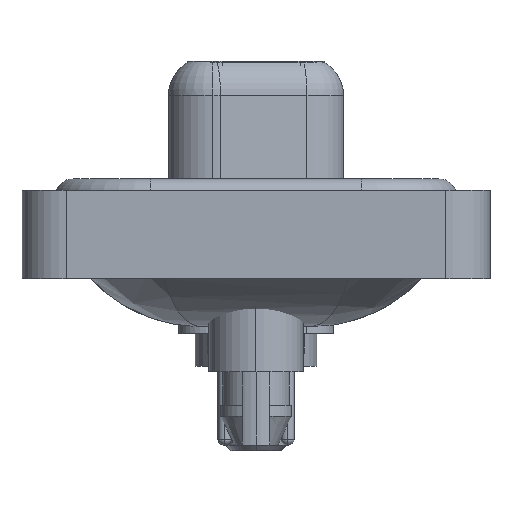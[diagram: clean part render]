
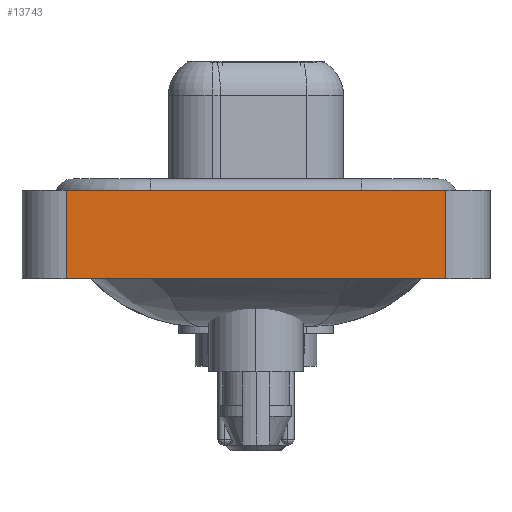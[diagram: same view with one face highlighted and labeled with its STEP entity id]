
A CAD part, left-side view. The second image highlights one B-rep face of the part: STEP entity #13743.
In plain terms, the highlighted planar face has unit normal (-1, 0, 0).
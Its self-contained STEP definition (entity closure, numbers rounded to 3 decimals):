
#519 = CARTESIAN_POINT ( 'NONE',  ( -7.25, -8.55, -3.6 ) ) ;
#941 = DIRECTION ( 'NONE',  ( 0., -1., 0. ) ) ;
#1468 = CARTESIAN_POINT ( 'NONE',  ( -7.25, -8.55, -3.6 ) ) ;
#1543 = EDGE_LOOP ( 'NONE', ( #17771, #7898, #10670, #3893 ) ) ;
#1933 = CARTESIAN_POINT ( 'NONE',  ( -7.25, -8.55, 0.4 ) ) ;
#3010 = EDGE_CURVE ( 'NONE', #9094, #14878, #14602, .T. ) ;
#3022 = AXIS2_PLACEMENT_3D ( 'NONE', #519, #16565, #19919 ) ;
#3397 = VECTOR ( 'NONE', #9768, 1000. ) ;
#3559 = PLANE ( 'NONE',  #3022 ) ;
#3672 = CARTESIAN_POINT ( 'NONE',  ( -7.25, -8.55, -3.6 ) ) ;
#3893 = ORIENTED_EDGE ( 'NONE', *, *, #6115, .T. ) ;
#4909 = LINE ( 'NONE', #1468, #3397 ) ;
#5332 = EDGE_CURVE ( 'NONE', #20415, #6546, #4909, .T. ) ;
#6093 = EDGE_CURVE ( 'NONE', #14878, #6546, #12459, .T. ) ;
#6115 = EDGE_CURVE ( 'NONE', #9094, #20415, #18401, .T. ) ;
#6188 = VECTOR ( 'NONE', #14391, 1000. ) ;
#6546 = VERTEX_POINT ( 'NONE', #15662 ) ;
#7898 = ORIENTED_EDGE ( 'NONE', *, *, #6093, .F. ) ;
#9094 = VERTEX_POINT ( 'NONE', #14737 ) ;
#9768 = DIRECTION ( 'NONE',  ( 0., 0., 1. ) ) ;
#10670 = ORIENTED_EDGE ( 'NONE', *, *, #3010, .F. ) ;
#12459 = LINE ( 'NONE', #1933, #17845 ) ;
#13743 = ADVANCED_FACE ( 'NONE', ( #19805 ), #3559, .T. ) ;
#14391 = DIRECTION ( 'NONE',  ( 0., -1., 0. ) ) ;
#14602 = LINE ( 'NONE', #16230, #18482 ) ;
#14737 = CARTESIAN_POINT ( 'NONE',  ( -7.25, 8.55, -3.6 ) ) ;
#14878 = VERTEX_POINT ( 'NONE', #21036 ) ;
#15662 = CARTESIAN_POINT ( 'NONE',  ( -7.25, -8.55, 0.4 ) ) ;
#16230 = CARTESIAN_POINT ( 'NONE',  ( -7.25, 8.55, -3.6 ) ) ;
#16565 = DIRECTION ( 'NONE',  ( -1., 0., 0. ) ) ;
#17747 = DIRECTION ( 'NONE',  ( 0., 0., 1. ) ) ;
#17771 = ORIENTED_EDGE ( 'NONE', *, *, #5332, .T. ) ;
#17820 = CARTESIAN_POINT ( 'NONE',  ( -7.25, -8.55, -3.6 ) ) ;
#17845 = VECTOR ( 'NONE', #941, 1000. ) ;
#18401 = LINE ( 'NONE', #3672, #6188 ) ;
#18482 = VECTOR ( 'NONE', #17747, 1000. ) ;
#19805 = FACE_OUTER_BOUND ( 'NONE', #1543, .T. ) ;
#19919 = DIRECTION ( 'NONE',  ( 0., 0., 1. ) ) ;
#20415 = VERTEX_POINT ( 'NONE', #17820 ) ;
#21036 = CARTESIAN_POINT ( 'NONE',  ( -7.25, 8.55, 0.4 ) ) ;
